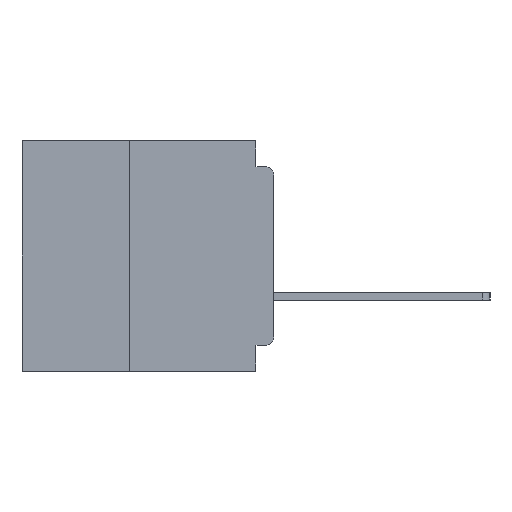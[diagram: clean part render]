
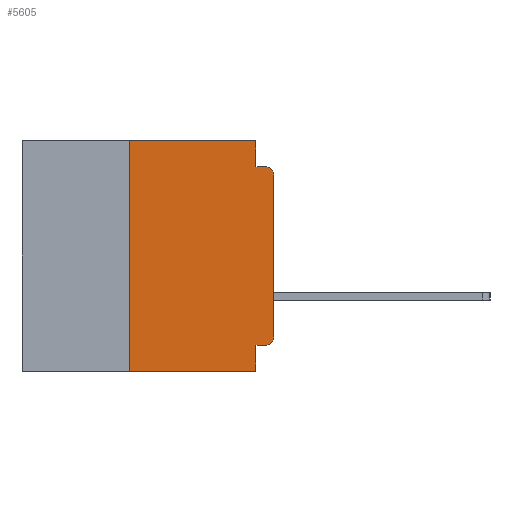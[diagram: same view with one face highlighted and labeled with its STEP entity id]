
A CAD part, left-side view. The second image highlights one B-rep face of the part: STEP entity #5605.
In plain terms, the highlighted planar face has unit normal (-1, 0, 0).
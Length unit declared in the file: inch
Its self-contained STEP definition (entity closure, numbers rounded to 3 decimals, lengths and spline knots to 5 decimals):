
#1619 = VECTOR ( 'NONE', #28087, 39.37008 ) ;
#2193 = EDGE_CURVE ( 'NONE', #10073, #27000, #34686, .T. ) ;
#2214 = CARTESIAN_POINT ( 'NONE',  ( 0., 0.031, -0.4 ) ) ;
#2381 = VERTEX_POINT ( 'NONE', #10683 ) ;
#2836 = DIRECTION ( 'NONE',  ( -1., 0., 0. ) ) ;
#3159 = CARTESIAN_POINT ( 'NONE',  ( 0., 0., -0.045 ) ) ;
#3817 = EDGE_CURVE ( 'NONE', #29826, #2381, #39573, .T. ) ;
#4032 = VERTEX_POINT ( 'NONE', #26252 ) ;
#4968 = CARTESIAN_POINT ( 'NONE',  ( 0., 0.031, 0. ) ) ;
#5605 = ADVANCED_FACE ( 'NONE', ( #15243 ), #28095, .F. ) ;
#6425 = EDGE_CURVE ( 'NONE', #4032, #14294, #40944, .T. ) ;
#7341 = CARTESIAN_POINT ( 'NONE',  ( 0., 0.031, -0.045 ) ) ;
#7373 = VECTOR ( 'NONE', #22825, 39.37008 ) ;
#8913 = DIRECTION ( 'NONE',  ( 0., 0., -1. ) ) ;
#9234 = CIRCLE ( 'NONE', #34899, 0.015 ) ;
#9352 = ORIENTED_EDGE ( 'NONE', *, *, #28666, .T. ) ;
#10073 = VERTEX_POINT ( 'NONE', #7341 ) ;
#10683 = CARTESIAN_POINT ( 'NONE',  ( 0., 0.031, -0.4 ) ) ;
#11877 = VECTOR ( 'NONE', #27937, 39.37008 ) ;
#13167 = EDGE_CURVE ( 'NONE', #15244, #29826, #39887, .T. ) ;
#14294 = VERTEX_POINT ( 'NONE', #36352 ) ;
#14763 = VECTOR ( 'NONE', #8913, 39.37008 ) ;
#15137 = ORIENTED_EDGE ( 'NONE', *, *, #36366, .F. ) ;
#15152 = VECTOR ( 'NONE', #16608, 39.37008 ) ;
#15243 = FACE_OUTER_BOUND ( 'NONE', #34006, .T. ) ;
#15244 = VERTEX_POINT ( 'NONE', #32280 ) ;
#15261 = DIRECTION ( 'NONE',  ( -1., 0., 0. ) ) ;
#15285 = ORIENTED_EDGE ( 'NONE', *, *, #2193, .F. ) ;
#15931 = CARTESIAN_POINT ( 'NONE',  ( 0., 0.437, 0. ) ) ;
#16449 = ORIENTED_EDGE ( 'NONE', *, *, #16537, .T. ) ;
#16537 = EDGE_CURVE ( 'NONE', #4032, #2381, #32420, .T. ) ;
#16608 = DIRECTION ( 'NONE',  ( 0., -1., 0. ) ) ;
#16856 = EDGE_CURVE ( 'NONE', #25522, #39403, #19263, .T. ) ;
#17942 = ORIENTED_EDGE ( 'NONE', *, *, #23650, .T. ) ;
#19263 = LINE ( 'NONE', #37599, #1619 ) ;
#20215 = CARTESIAN_POINT ( 'NONE',  ( 0., 0., -0.06 ) ) ;
#20452 = DIRECTION ( 'NONE',  ( 0., 1., 0. ) ) ;
#21328 = AXIS2_PLACEMENT_3D ( 'NONE', #34649, #15261, #37864 ) ;
#22635 = CARTESIAN_POINT ( 'NONE',  ( 0., 0.015, -0.06 ) ) ;
#22825 = DIRECTION ( 'NONE',  ( 0., 0., 1. ) ) ;
#23400 = CARTESIAN_POINT ( 'NONE',  ( 0., 0., -0.34 ) ) ;
#23650 = EDGE_CURVE ( 'NONE', #39403, #27000, #9234, .T. ) ;
#24860 = CARTESIAN_POINT ( 'NONE',  ( 0., 0.437, 0. ) ) ;
#25522 = VERTEX_POINT ( 'NONE', #23400 ) ;
#25705 = ORIENTED_EDGE ( 'NONE', *, *, #3817, .F. ) ;
#25885 = DIRECTION ( 'NONE',  ( 0., 0., -1. ) ) ;
#26239 = CARTESIAN_POINT ( 'NONE',  ( 0., 0.015, -0.045 ) ) ;
#26252 = CARTESIAN_POINT ( 'NONE',  ( 0., 0.25, -0.4 ) ) ;
#27000 = VERTEX_POINT ( 'NONE', #26239 ) ;
#27666 = CIRCLE ( 'NONE', #21328, 0.015 ) ;
#27937 = DIRECTION ( 'NONE',  ( 0., 0., -1. ) ) ;
#28087 = DIRECTION ( 'NONE',  ( 0., 0., 1. ) ) ;
#28095 = PLANE ( 'NONE',  #37326 ) ;
#28236 = LINE ( 'NONE', #4968, #11877 ) ;
#28666 = EDGE_CURVE ( 'NONE', #15244, #25522, #27666, .T. ) ;
#29826 = VERTEX_POINT ( 'NONE', #30448 ) ;
#30448 = CARTESIAN_POINT ( 'NONE',  ( 0., 0.031, -0.355 ) ) ;
#30768 = CARTESIAN_POINT ( 'NONE',  ( 0., 0.031, 0. ) ) ;
#31030 = ORIENTED_EDGE ( 'NONE', *, *, #13167, .F. ) ;
#31331 = DIRECTION ( 'NONE',  ( 0., 0., -1. ) ) ;
#31339 = VECTOR ( 'NONE', #41771, 39.37008 ) ;
#31363 = VECTOR ( 'NONE', #20452, 39.37008 ) ;
#32009 = ORIENTED_EDGE ( 'NONE', *, *, #16856, .T. ) ;
#32280 = CARTESIAN_POINT ( 'NONE',  ( 0., 0.015, -0.355 ) ) ;
#32420 = LINE ( 'NONE', #32892, #15152 ) ;
#32892 = CARTESIAN_POINT ( 'NONE',  ( 0., 0.437, -0.4 ) ) ;
#34006 = EDGE_LOOP ( 'NONE', ( #32009, #17942, #15285, #15137, #36944, #42217, #16449, #25705, #31030, #9352 ) ) ;
#34403 = DIRECTION ( 'NONE',  ( 1., 0., 0. ) ) ;
#34649 = CARTESIAN_POINT ( 'NONE',  ( 0., 0.015, -0.34 ) ) ;
#34686 = LINE ( 'NONE', #3159, #42220 ) ;
#34899 = AXIS2_PLACEMENT_3D ( 'NONE', #22635, #2836, #25885 ) ;
#35479 = EDGE_CURVE ( 'NONE', #14294, #39558, #39864, .T. ) ;
#35843 = DIRECTION ( 'NONE',  ( 0., -1., 0. ) ) ;
#36352 = CARTESIAN_POINT ( 'NONE',  ( 0., 0.25, 0. ) ) ;
#36366 = EDGE_CURVE ( 'NONE', #39558, #10073, #28236, .T. ) ;
#36434 = CARTESIAN_POINT ( 'NONE',  ( 0., 0., -0.355 ) ) ;
#36944 = ORIENTED_EDGE ( 'NONE', *, *, #35479, .F. ) ;
#37326 = AXIS2_PLACEMENT_3D ( 'NONE', #24860, #34403, #31331 ) ;
#37599 = CARTESIAN_POINT ( 'NONE',  ( 0., 0., 0. ) ) ;
#37864 = DIRECTION ( 'NONE',  ( 0., 0., -1. ) ) ;
#39403 = VERTEX_POINT ( 'NONE', #20215 ) ;
#39558 = VERTEX_POINT ( 'NONE', #30768 ) ;
#39573 = LINE ( 'NONE', #2214, #14763 ) ;
#39864 = LINE ( 'NONE', #15931, #31339 ) ;
#39887 = LINE ( 'NONE', #36434, #31363 ) ;
#40944 = LINE ( 'NONE', #42059, #7373 ) ;
#41771 = DIRECTION ( 'NONE',  ( 0., -1., 0. ) ) ;
#42059 = CARTESIAN_POINT ( 'NONE',  ( 0., 0.25, -0.4 ) ) ;
#42217 = ORIENTED_EDGE ( 'NONE', *, *, #6425, .F. ) ;
#42220 = VECTOR ( 'NONE', #35843, 39.37008 ) ;
